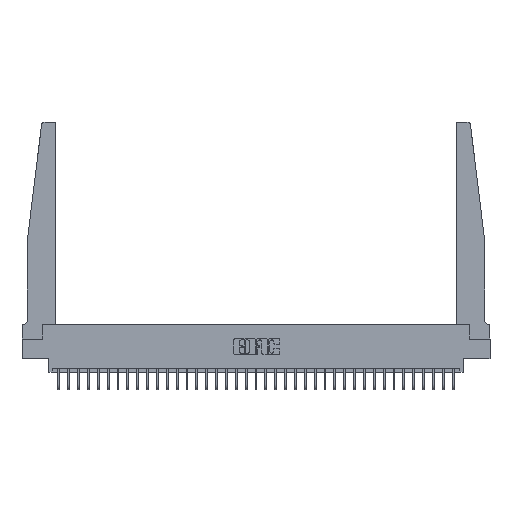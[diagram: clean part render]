
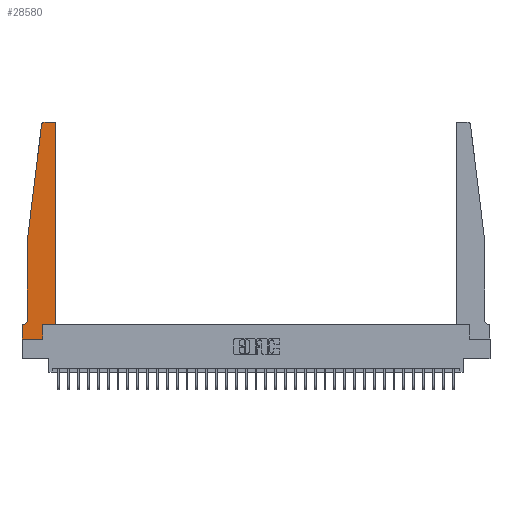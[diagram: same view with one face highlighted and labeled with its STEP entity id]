
A CAD part, top view. The second image highlights one B-rep face of the part: STEP entity #28580.
In plain terms, the highlighted planar face has unit normal (0, 0, 1).
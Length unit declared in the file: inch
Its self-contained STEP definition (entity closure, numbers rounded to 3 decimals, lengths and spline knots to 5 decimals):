
#73 = ORIENTED_EDGE ( 'NONE', *, *, #9776, .T. ) ;
#191 = DIRECTION ( 'NONE',  ( 0., 1., 0. ) ) ;
#409 = CIRCLE ( 'NONE', #3861, 0.03 ) ;
#1356 = AXIS2_PLACEMENT_3D ( 'NONE', #7970, #31456, #3054 ) ;
#1374 = DIRECTION ( 'NONE',  ( 0., -1., 0. ) ) ;
#1618 = VERTEX_POINT ( 'NONE', #9542 ) ;
#1957 = LINE ( 'NONE', #10153, #22298 ) ;
#2765 = CARTESIAN_POINT ( 'NONE',  ( 0.425, 0.18, 0.37 ) ) ;
#2825 = ORIENTED_EDGE ( 'NONE', *, *, #7453, .T. ) ;
#2934 = ORIENTED_EDGE ( 'NONE', *, *, #3562, .T. ) ;
#3054 = DIRECTION ( 'NONE',  ( -1., 0., 0. ) ) ;
#3562 = EDGE_CURVE ( 'NONE', #11749, #33410, #30951, .T. ) ;
#3593 = CARTESIAN_POINT ( 'NONE',  ( 0., 0.1875, 0.37 ) ) ;
#3842 = VERTEX_POINT ( 'NONE', #3593 ) ;
#3861 = AXIS2_PLACEMENT_3D ( 'NONE', #23025, #4608, #9910 ) ;
#3907 = EDGE_CURVE ( 'NONE', #3842, #9815, #29742, .T. ) ;
#4387 = LINE ( 'NONE', #6469, #28751 ) ;
#4608 = DIRECTION ( 'NONE',  ( 0., 0., 1. ) ) ;
#5218 = CARTESIAN_POINT ( 'NONE',  ( 0.27653, 2.72, 0.37 ) ) ;
#5375 = PLANE ( 'NONE',  #22919 ) ;
#5575 = CARTESIAN_POINT ( 'NONE',  ( 0.425, 0.18, 0.37 ) ) ;
#5604 = CARTESIAN_POINT ( 'NONE',  ( 0., 0.1875, 0.37 ) ) ;
#6150 = VERTEX_POINT ( 'NONE', #5575 ) ;
#6469 = CARTESIAN_POINT ( 'NONE',  ( 0.065, 1.25, 0.37 ) ) ;
#6479 = ORIENTED_EDGE ( 'NONE', *, *, #18951, .T. ) ;
#7002 = VECTOR ( 'NONE', #25433, 39.37008 ) ;
#7453 = EDGE_CURVE ( 'NONE', #21008, #3842, #14819, .T. ) ;
#7717 = CARTESIAN_POINT ( 'NONE',  ( 0.425, 0.18, 0.37 ) ) ;
#7970 = CARTESIAN_POINT ( 'NONE',  ( 0.015, 0.2375, 0.37 ) ) ;
#8026 = FACE_OUTER_BOUND ( 'NONE', #14128, .T. ) ;
#8580 = LINE ( 'NONE', #2765, #18712 ) ;
#8585 = DIRECTION ( 'NONE',  ( -1., 0., 0. ) ) ;
#9105 = VECTOR ( 'NONE', #8585, 39.37008 ) ;
#9370 = VECTOR ( 'NONE', #191, 39.37008 ) ;
#9500 = EDGE_CURVE ( 'NONE', #18203, #29375, #1957, .T. ) ;
#9542 = CARTESIAN_POINT ( 'NONE',  ( 0.425, 2.72, 0.37 ) ) ;
#9776 = EDGE_CURVE ( 'NONE', #9815, #11749, #32403, .T. ) ;
#9815 = VERTEX_POINT ( 'NONE', #30924 ) ;
#9885 = DIRECTION ( 'NONE',  ( 1., 0., 0. ) ) ;
#9910 = DIRECTION ( 'NONE',  ( 1., 0., 0. ) ) ;
#9911 = CARTESIAN_POINT ( 'NONE',  ( 0.2605, 0.18, 0.37 ) ) ;
#10153 = CARTESIAN_POINT ( 'NONE',  ( 0.25, 2.75, 0.37 ) ) ;
#10345 = VERTEX_POINT ( 'NONE', #30404 ) ;
#10934 = ORIENTED_EDGE ( 'NONE', *, *, #19865, .T. ) ;
#11057 = LINE ( 'NONE', #26306, #20413 ) ;
#11749 = VERTEX_POINT ( 'NONE', #31559 ) ;
#12347 = ORIENTED_EDGE ( 'NONE', *, *, #14491, .T. ) ;
#12847 = DIRECTION ( 'NONE',  ( -1., 0., 0. ) ) ;
#13130 = DIRECTION ( 'NONE',  ( 0., 0., 1. ) ) ;
#13468 = DIRECTION ( 'NONE',  ( -0.122, -0.992, 0. ) ) ;
#13926 = EDGE_CURVE ( 'NONE', #33410, #6150, #8580, .T. ) ;
#14128 = EDGE_LOOP ( 'NONE', ( #29751, #23591, #19526, #10934, #12347, #2825, #22079, #73, #2934, #32579, #6479, #29730 ) ) ;
#14491 = EDGE_CURVE ( 'NONE', #10345, #21008, #26261, .T. ) ;
#14577 = CARTESIAN_POINT ( 'NONE',  ( 0.27653, 2.75, 0.37 ) ) ;
#14819 = LINE ( 'NONE', #28967, #9105 ) ;
#16238 = LINE ( 'NONE', #7717, #9370 ) ;
#17385 = CARTESIAN_POINT ( 'NONE',  ( 0.395, 2.75, 0.37 ) ) ;
#17542 = EDGE_CURVE ( 'NONE', #31542, #29315, #11057, .T. ) ;
#17882 = CARTESIAN_POINT ( 'NONE',  ( 0., 0., 0.37 ) ) ;
#18203 = VERTEX_POINT ( 'NONE', #17385 ) ;
#18712 = VECTOR ( 'NONE', #31376, 39.37008 ) ;
#18783 = CARTESIAN_POINT ( 'NONE',  ( 0.24675, 2.72367, 0.37 ) ) ;
#18901 = CIRCLE ( 'NONE', #20930, 0.03 ) ;
#18951 = EDGE_CURVE ( 'NONE', #6150, #1618, #16238, .T. ) ;
#19243 = CARTESIAN_POINT ( 'NONE',  ( 0.015, 0.1875, 0.37 ) ) ;
#19526 = ORIENTED_EDGE ( 'NONE', *, *, #17542, .T. ) ;
#19865 = EDGE_CURVE ( 'NONE', #29315, #10345, #4387, .T. ) ;
#20413 = VECTOR ( 'NONE', #13468, 39.37008 ) ;
#20930 = AXIS2_PLACEMENT_3D ( 'NONE', #5218, #28627, #23555 ) ;
#21008 = VERTEX_POINT ( 'NONE', #19243 ) ;
#21317 = CARTESIAN_POINT ( 'NONE',  ( 0.2605, 0.18, 0.37 ) ) ;
#22079 = ORIENTED_EDGE ( 'NONE', *, *, #3907, .T. ) ;
#22298 = VECTOR ( 'NONE', #12847, 39.37008 ) ;
#22331 = EDGE_CURVE ( 'NONE', #1618, #18203, #409, .T. ) ;
#22919 = AXIS2_PLACEMENT_3D ( 'NONE', #5604, #13130, #28994 ) ;
#23025 = CARTESIAN_POINT ( 'NONE',  ( 0.395, 2.72, 0.37 ) ) ;
#23039 = VECTOR ( 'NONE', #9885, 39.37008 ) ;
#23555 = DIRECTION ( 'NONE',  ( 1., 0., 0. ) ) ;
#23591 = ORIENTED_EDGE ( 'NONE', *, *, #30114, .T. ) ;
#24941 = VECTOR ( 'NONE', #31489, 39.37008 ) ;
#25433 = DIRECTION ( 'NONE',  ( 0., -1., 0. ) ) ;
#26261 = CIRCLE ( 'NONE', #1356, 0.05 ) ;
#26306 = CARTESIAN_POINT ( 'NONE',  ( 0.065, 1.25, 0.37 ) ) ;
#27807 = CARTESIAN_POINT ( 'NONE',  ( 0.065, 1.25, 0.37 ) ) ;
#28580 = ADVANCED_FACE ( 'NONE', ( #8026 ), #5375, .T. ) ;
#28627 = DIRECTION ( 'NONE',  ( 0., 0., 1. ) ) ;
#28751 = VECTOR ( 'NONE', #1374, 39.37008 ) ;
#28967 = CARTESIAN_POINT ( 'NONE',  ( 0.065, 0.1875, 0.37 ) ) ;
#28994 = DIRECTION ( 'NONE',  ( 1., 0., 0. ) ) ;
#29315 = VERTEX_POINT ( 'NONE', #27807 ) ;
#29375 = VERTEX_POINT ( 'NONE', #14577 ) ;
#29730 = ORIENTED_EDGE ( 'NONE', *, *, #22331, .T. ) ;
#29742 = LINE ( 'NONE', #31028, #7002 ) ;
#29751 = ORIENTED_EDGE ( 'NONE', *, *, #9500, .T. ) ;
#30114 = EDGE_CURVE ( 'NONE', #29375, #31542, #18901, .T. ) ;
#30404 = CARTESIAN_POINT ( 'NONE',  ( 0.065, 0.2375, 0.37 ) ) ;
#30924 = CARTESIAN_POINT ( 'NONE',  ( 0., 0., 0.37 ) ) ;
#30951 = LINE ( 'NONE', #21317, #24941 ) ;
#31028 = CARTESIAN_POINT ( 'NONE',  ( 0., 0., 0.37 ) ) ;
#31376 = DIRECTION ( 'NONE',  ( 1., 0., 0. ) ) ;
#31456 = DIRECTION ( 'NONE',  ( 0., 0., -1. ) ) ;
#31489 = DIRECTION ( 'NONE',  ( 0., 1., 0. ) ) ;
#31542 = VERTEX_POINT ( 'NONE', #18783 ) ;
#31559 = CARTESIAN_POINT ( 'NONE',  ( 0.2605, 0., 0.37 ) ) ;
#32403 = LINE ( 'NONE', #17882, #23039 ) ;
#32579 = ORIENTED_EDGE ( 'NONE', *, *, #13926, .T. ) ;
#33410 = VERTEX_POINT ( 'NONE', #9911 ) ;
